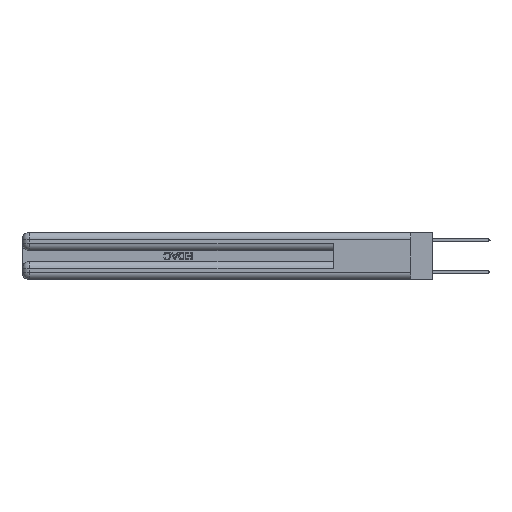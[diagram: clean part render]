
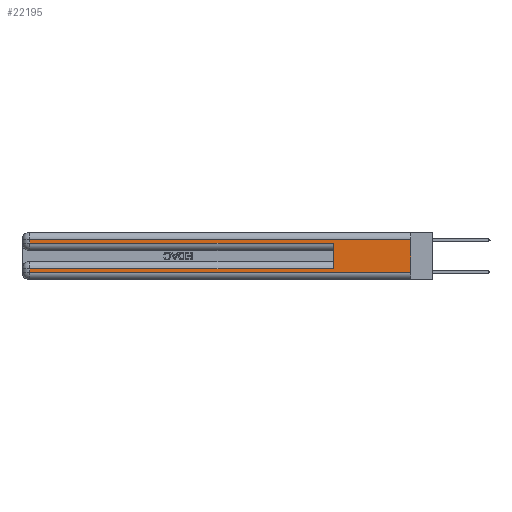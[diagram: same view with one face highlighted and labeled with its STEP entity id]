
A CAD part, left-side view. The second image highlights one B-rep face of the part: STEP entity #22195.
In plain terms, the highlighted planar face has unit normal (-1, 0, 0).
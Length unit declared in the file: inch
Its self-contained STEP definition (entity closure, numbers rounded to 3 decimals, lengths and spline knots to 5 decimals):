
#1968 = LINE ( 'NONE', #8143, #15726 ) ;
#2528 = LINE ( 'NONE', #33083, #16281 ) ;
#4159 = CARTESIAN_POINT ( 'NONE',  ( 0., 0.6, 0.285 ) ) ;
#4288 = VECTOR ( 'NONE', #29818, 39.37008 ) ;
#4471 = VERTEX_POINT ( 'NONE', #12273 ) ;
#5682 = CARTESIAN_POINT ( 'NONE',  ( 0., 0., 0.06 ) ) ;
#6176 = CARTESIAN_POINT ( 'NONE',  ( 0., 0., 0.31 ) ) ;
#6669 = ORIENTED_EDGE ( 'NONE', *, *, #8488, .T. ) ;
#7721 = ORIENTED_EDGE ( 'NONE', *, *, #26416, .T. ) ;
#8143 = CARTESIAN_POINT ( 'NONE',  ( 0., 0., 0.06 ) ) ;
#8178 = EDGE_LOOP ( 'NONE', ( #16122, #6669, #29413, #7721, #22528, #11074, #21900, #25338 ) ) ;
#8488 = EDGE_CURVE ( 'NONE', #20127, #12281, #27373, .T. ) ;
#8655 = EDGE_CURVE ( 'NONE', #4471, #21204, #18350, .T. ) ;
#8718 = DIRECTION ( 'NONE',  ( 0., 0., -1. ) ) ;
#8750 = CARTESIAN_POINT ( 'NONE',  ( 0., 2.94, 0.31 ) ) ;
#8947 = DIRECTION ( 'NONE',  ( 0., 1., 0. ) ) ;
#9749 = PLANE ( 'NONE',  #16259 ) ;
#10761 = EDGE_CURVE ( 'NONE', #18543, #21962, #1968, .T. ) ;
#11074 = ORIENTED_EDGE ( 'NONE', *, *, #14837, .T. ) ;
#11364 = CARTESIAN_POINT ( 'NONE',  ( 0., 2.94, 0.285 ) ) ;
#12255 = CARTESIAN_POINT ( 'NONE',  ( 0., 0.6, 0.145 ) ) ;
#12273 = CARTESIAN_POINT ( 'NONE',  ( 0., 0.6, 0.085 ) ) ;
#12281 = VERTEX_POINT ( 'NONE', #8750 ) ;
#12508 = DIRECTION ( 'NONE',  ( 1., 0., 0. ) ) ;
#12664 = DIRECTION ( 'NONE',  ( 0., -1., 0. ) ) ;
#13366 = DIRECTION ( 'NONE',  ( 0., 1., 0. ) ) ;
#13832 = DIRECTION ( 'NONE',  ( 0., 0., -1. ) ) ;
#14837 = EDGE_CURVE ( 'NONE', #4471, #26905, #19047, .T. ) ;
#15474 = LINE ( 'NONE', #19281, #29129 ) ;
#15726 = VECTOR ( 'NONE', #27224, 39.37008 ) ;
#16122 = ORIENTED_EDGE ( 'NONE', *, *, #33918, .F. ) ;
#16259 = AXIS2_PLACEMENT_3D ( 'NONE', #26127, #12508, #31556 ) ;
#16281 = VECTOR ( 'NONE', #8718, 39.37008 ) ;
#16569 = CARTESIAN_POINT ( 'NONE',  ( 0., 0., 0.31 ) ) ;
#16647 = VECTOR ( 'NONE', #28612, 39.37008 ) ;
#18117 = CARTESIAN_POINT ( 'NONE',  ( 0., 0., 0.285 ) ) ;
#18202 = VECTOR ( 'NONE', #13366, 39.37008 ) ;
#18310 = EDGE_CURVE ( 'NONE', #12281, #23164, #15474, .T. ) ;
#18350 = LINE ( 'NONE', #12255, #16647 ) ;
#18543 = VERTEX_POINT ( 'NONE', #34480 ) ;
#18928 = CARTESIAN_POINT ( 'NONE',  ( 0., 2.94, 0.37 ) ) ;
#19047 = LINE ( 'NONE', #29586, #18202 ) ;
#19281 = CARTESIAN_POINT ( 'NONE',  ( 0., 2.94, 0.37 ) ) ;
#20047 = VECTOR ( 'NONE', #8947, 39.37008 ) ;
#20127 = VERTEX_POINT ( 'NONE', #16569 ) ;
#21204 = VERTEX_POINT ( 'NONE', #4159 ) ;
#21900 = ORIENTED_EDGE ( 'NONE', *, *, #26576, .T. ) ;
#21962 = VERTEX_POINT ( 'NONE', #5682 ) ;
#22195 = ADVANCED_FACE ( 'NONE', ( #35311 ), #9749, .F. ) ;
#22528 = ORIENTED_EDGE ( 'NONE', *, *, #8655, .F. ) ;
#23140 = VECTOR ( 'NONE', #12664, 39.37008 ) ;
#23164 = VERTEX_POINT ( 'NONE', #11364 ) ;
#25338 = ORIENTED_EDGE ( 'NONE', *, *, #10761, .T. ) ;
#26127 = CARTESIAN_POINT ( 'NONE',  ( 0., 0., 0.37 ) ) ;
#26416 = EDGE_CURVE ( 'NONE', #23164, #21204, #31240, .T. ) ;
#26576 = EDGE_CURVE ( 'NONE', #26905, #18543, #27853, .T. ) ;
#26905 = VERTEX_POINT ( 'NONE', #28604 ) ;
#27224 = DIRECTION ( 'NONE',  ( 0., -1., 0. ) ) ;
#27373 = LINE ( 'NONE', #6176, #20047 ) ;
#27853 = LINE ( 'NONE', #18928, #4288 ) ;
#28604 = CARTESIAN_POINT ( 'NONE',  ( 0., 2.94, 0.085 ) ) ;
#28612 = DIRECTION ( 'NONE',  ( 0., 0., 1. ) ) ;
#29129 = VECTOR ( 'NONE', #13832, 39.37008 ) ;
#29413 = ORIENTED_EDGE ( 'NONE', *, *, #18310, .T. ) ;
#29586 = CARTESIAN_POINT ( 'NONE',  ( 0., 0., 0.085 ) ) ;
#29818 = DIRECTION ( 'NONE',  ( 0., 0., -1. ) ) ;
#31240 = LINE ( 'NONE', #18117, #23140 ) ;
#31556 = DIRECTION ( 'NONE',  ( 0., 0., -1. ) ) ;
#33083 = CARTESIAN_POINT ( 'NONE',  ( 0., 0., 0.37 ) ) ;
#33918 = EDGE_CURVE ( 'NONE', #20127, #21962, #2528, .T. ) ;
#34480 = CARTESIAN_POINT ( 'NONE',  ( 0., 2.94, 0.06 ) ) ;
#35311 = FACE_OUTER_BOUND ( 'NONE', #8178, .T. ) ;
